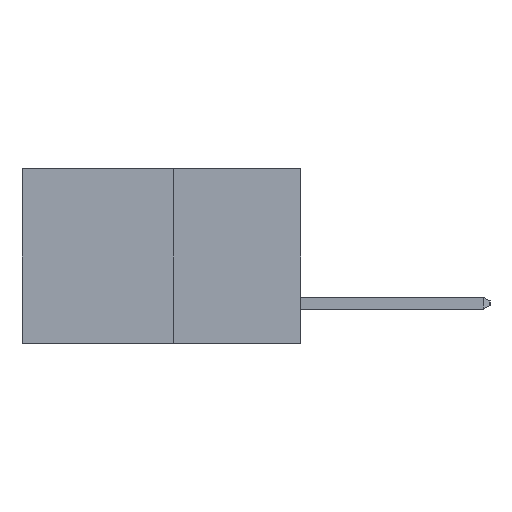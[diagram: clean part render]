
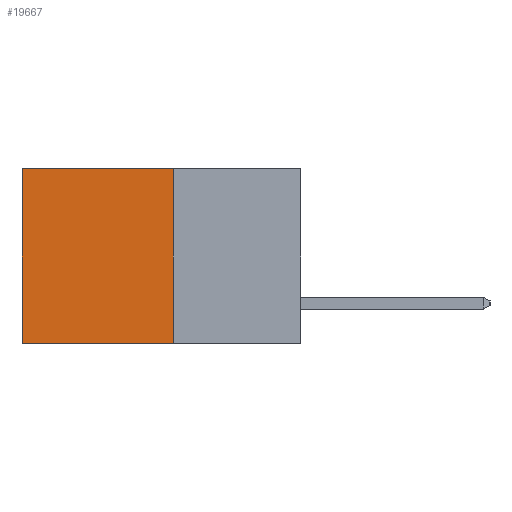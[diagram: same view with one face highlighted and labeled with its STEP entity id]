
A CAD part, left-side view. The second image highlights one B-rep face of the part: STEP entity #19667.
In plain terms, the highlighted planar face has unit normal (-1, 0, 0).
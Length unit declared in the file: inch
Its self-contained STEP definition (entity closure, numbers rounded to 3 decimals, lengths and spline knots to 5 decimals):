
#55 = LINE ( 'NONE', #5962, #4703 ) ;
#113 = DIRECTION ( 'NONE',  ( 1., 0., 0. ) ) ;
#1372 = VERTEX_POINT ( 'NONE', #2996 ) ;
#2064 = ORIENTED_EDGE ( 'NONE', *, *, #21789, .F. ) ;
#2996 = CARTESIAN_POINT ( 'NONE',  ( 0.277, 0.59, -0.37 ) ) ;
#3166 = VERTEX_POINT ( 'NONE', #8852 ) ;
#4463 = VECTOR ( 'NONE', #11220, 39.37008 ) ;
#4703 = VECTOR ( 'NONE', #19795, 39.37008 ) ;
#4827 = VERTEX_POINT ( 'NONE', #16139 ) ;
#4894 = VECTOR ( 'NONE', #15722, 39.37008 ) ;
#4902 = EDGE_LOOP ( 'NONE', ( #13816, #2064, #7379, #6608 ) ) ;
#5955 = LINE ( 'NONE', #7116, #4894 ) ;
#5962 = CARTESIAN_POINT ( 'NONE',  ( 0.277, 0.27, -0.37 ) ) ;
#6608 = ORIENTED_EDGE ( 'NONE', *, *, #10377, .T. ) ;
#7116 = CARTESIAN_POINT ( 'NONE',  ( 0.277, 0.27, -0.37 ) ) ;
#7379 = ORIENTED_EDGE ( 'NONE', *, *, #17813, .F. ) ;
#8852 = CARTESIAN_POINT ( 'NONE',  ( 0.277, 0.27, -0.37 ) ) ;
#10377 = EDGE_CURVE ( 'NONE', #15283, #4827, #17619, .T. ) ;
#10498 = CARTESIAN_POINT ( 'NONE',  ( 0.277, 0.27, -0.37 ) ) ;
#11220 = DIRECTION ( 'NONE',  ( 0., 0., -1. ) ) ;
#11502 = DIRECTION ( 'NONE',  ( 0., 1., 0. ) ) ;
#11608 = FACE_OUTER_BOUND ( 'NONE', #4902, .T. ) ;
#12265 = DIRECTION ( 'NONE',  ( 0., 0., -1. ) ) ;
#12939 = CARTESIAN_POINT ( 'NONE',  ( 0.277, 0.59, -0.37 ) ) ;
#13138 = CARTESIAN_POINT ( 'NONE',  ( 0.277, 0.27, 0. ) ) ;
#13203 = AXIS2_PLACEMENT_3D ( 'NONE', #10498, #113, #12265 ) ;
#13651 = LINE ( 'NONE', #12939, #4463 ) ;
#13816 = ORIENTED_EDGE ( 'NONE', *, *, #21178, .T. ) ;
#15283 = VERTEX_POINT ( 'NONE', #21468 ) ;
#15722 = DIRECTION ( 'NONE',  ( 0., 0., -1. ) ) ;
#16139 = CARTESIAN_POINT ( 'NONE',  ( 0.277, 0.59, 0. ) ) ;
#17089 = VECTOR ( 'NONE', #11502, 39.37008 ) ;
#17368 = PLANE ( 'NONE',  #13203 ) ;
#17619 = LINE ( 'NONE', #13138, #17089 ) ;
#17813 = EDGE_CURVE ( 'NONE', #15283, #3166, #5955, .T. ) ;
#19667 = ADVANCED_FACE ( 'NONE', ( #11608 ), #17368, .F. ) ;
#19795 = DIRECTION ( 'NONE',  ( 0., 1., 0. ) ) ;
#21178 = EDGE_CURVE ( 'NONE', #4827, #1372, #13651, .T. ) ;
#21468 = CARTESIAN_POINT ( 'NONE',  ( 0.277, 0.27, 0. ) ) ;
#21789 = EDGE_CURVE ( 'NONE', #3166, #1372, #55, .T. ) ;
